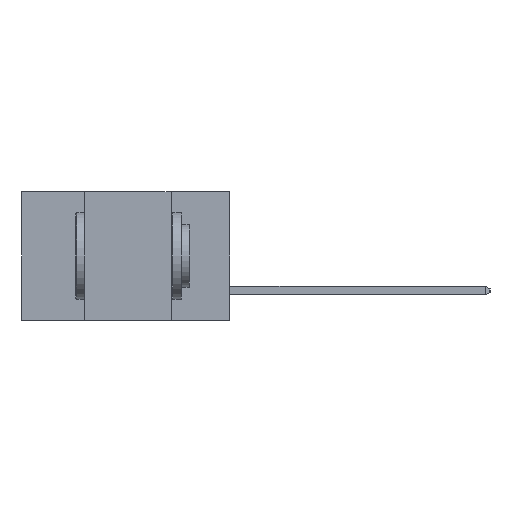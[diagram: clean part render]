
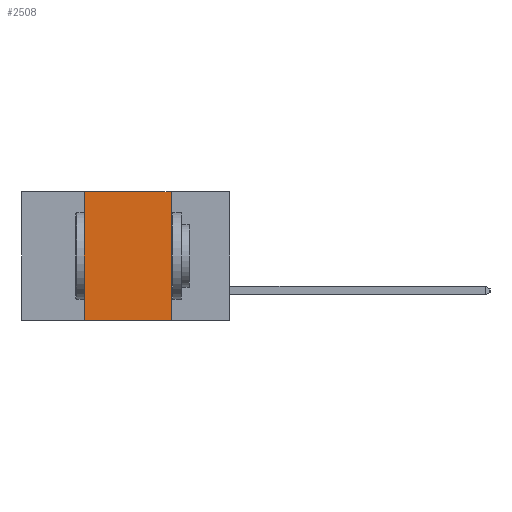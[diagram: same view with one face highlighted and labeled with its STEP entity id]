
A CAD part, left-side view. The second image highlights one B-rep face of the part: STEP entity #2508.
In plain terms, the highlighted planar face has unit normal (-1, 0, 0).
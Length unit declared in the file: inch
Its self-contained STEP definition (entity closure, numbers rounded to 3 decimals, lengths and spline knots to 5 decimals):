
#619 = VECTOR ( 'NONE', #11068, 39.37008 ) ;
#674 = VECTOR ( 'NONE', #13146, 39.37008 ) ;
#1225 = CARTESIAN_POINT ( 'NONE',  ( 0., 0.17, -0.37 ) ) ;
#1449 = DIRECTION ( 'NONE',  ( 0., -1., 0. ) ) ;
#1869 = ORIENTED_EDGE ( 'NONE', *, *, #6967, .F. ) ;
#2508 = ADVANCED_FACE ( 'NONE', ( #11594 ), #5030, .F. ) ;
#2567 = EDGE_LOOP ( 'NONE', ( #7233, #12293, #1869, #7548 ) ) ;
#4089 = VERTEX_POINT ( 'NONE', #1225 ) ;
#4740 = DIRECTION ( 'NONE',  ( 0., 0., -1. ) ) ;
#4755 = CARTESIAN_POINT ( 'NONE',  ( 0., 0.6, 0. ) ) ;
#4759 = DIRECTION ( 'NONE',  ( 1., 0., 0. ) ) ;
#4776 = CARTESIAN_POINT ( 'NONE',  ( 0., 0.6, 0. ) ) ;
#5015 = DIRECTION ( 'NONE',  ( 0., 0., 1. ) ) ;
#5030 = PLANE ( 'NONE',  #11331 ) ;
#6288 = EDGE_CURVE ( 'NONE', #10315, #4089, #11656, .T. ) ;
#6967 = EDGE_CURVE ( 'NONE', #10315, #12611, #11643, .T. ) ;
#7233 = ORIENTED_EDGE ( 'NONE', *, *, #8303, .F. ) ;
#7548 = ORIENTED_EDGE ( 'NONE', *, *, #6288, .T. ) ;
#7638 = EDGE_CURVE ( 'NONE', #12611, #10017, #13237, .T. ) ;
#8045 = CARTESIAN_POINT ( 'NONE',  ( 0., 0.42, -0.37 ) ) ;
#8204 = CARTESIAN_POINT ( 'NONE',  ( 0., 0.17, 0. ) ) ;
#8266 = VECTOR ( 'NONE', #1449, 39.37008 ) ;
#8303 = EDGE_CURVE ( 'NONE', #10017, #4089, #11418, .T. ) ;
#8929 = CARTESIAN_POINT ( 'NONE',  ( 0., 0.6, -0.37 ) ) ;
#9245 = CARTESIAN_POINT ( 'NONE',  ( 0., 0.42, 0. ) ) ;
#10017 = VERTEX_POINT ( 'NONE', #8204 ) ;
#10315 = VERTEX_POINT ( 'NONE', #13267 ) ;
#11068 = DIRECTION ( 'NONE',  ( 0., -1., 0. ) ) ;
#11331 = AXIS2_PLACEMENT_3D ( 'NONE', #4776, #4759, #4740 ) ;
#11361 = VECTOR ( 'NONE', #5015, 39.37008 ) ;
#11418 = LINE ( 'NONE', #12232, #674 ) ;
#11594 = FACE_OUTER_BOUND ( 'NONE', #2567, .T. ) ;
#11643 = LINE ( 'NONE', #8045, #11361 ) ;
#11656 = LINE ( 'NONE', #8929, #619 ) ;
#12232 = CARTESIAN_POINT ( 'NONE',  ( 0., 0.17, -0.37 ) ) ;
#12293 = ORIENTED_EDGE ( 'NONE', *, *, #7638, .F. ) ;
#12611 = VERTEX_POINT ( 'NONE', #9245 ) ;
#13146 = DIRECTION ( 'NONE',  ( 0., 0., -1. ) ) ;
#13237 = LINE ( 'NONE', #4755, #8266 ) ;
#13267 = CARTESIAN_POINT ( 'NONE',  ( 0., 0.42, -0.37 ) ) ;
